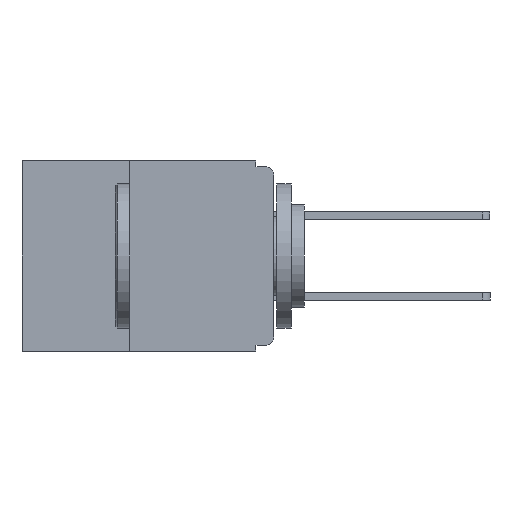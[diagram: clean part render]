
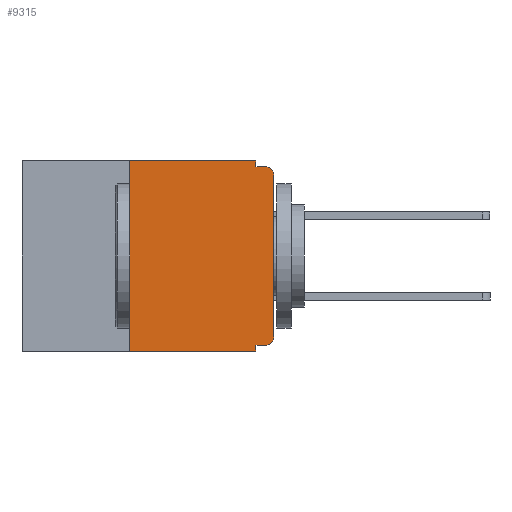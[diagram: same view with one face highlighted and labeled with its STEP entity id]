
A CAD part, left-side view. The second image highlights one B-rep face of the part: STEP entity #9315.
In plain terms, the highlighted planar face has unit normal (-1, 0, 0).
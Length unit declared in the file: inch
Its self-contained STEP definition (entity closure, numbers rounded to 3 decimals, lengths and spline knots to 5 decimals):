
#1121 = EDGE_CURVE ( 'NONE', #32581, #34202, #26190, .T. ) ;
#1328 = ORIENTED_EDGE ( 'NONE', *, *, #6280, .T. ) ;
#1453 = LINE ( 'NONE', #19023, #15636 ) ;
#1530 = EDGE_CURVE ( 'NONE', #34202, #16824, #20621, .T. ) ;
#2243 = ORIENTED_EDGE ( 'NONE', *, *, #1530, .F. ) ;
#2253 = LINE ( 'NONE', #21068, #15534 ) ;
#2695 = ORIENTED_EDGE ( 'NONE', *, *, #3785, .F. ) ;
#3785 = EDGE_CURVE ( 'NONE', #26825, #7777, #22980, .T. ) ;
#5232 = CARTESIAN_POINT ( 'NONE',  ( 0., 0.015, -0.01 ) ) ;
#5773 = ORIENTED_EDGE ( 'NONE', *, *, #33446, .F. ) ;
#6280 = EDGE_CURVE ( 'NONE', #29298, #16824, #17325, .T. ) ;
#6880 = CARTESIAN_POINT ( 'NONE',  ( 0., 0.031, -0.33 ) ) ;
#7129 = CIRCLE ( 'NONE', #20859, 0.015 ) ;
#7777 = VERTEX_POINT ( 'NONE', #15712 ) ;
#7837 = DIRECTION ( 'NONE',  ( 0., 0., -1. ) ) ;
#7987 = ORIENTED_EDGE ( 'NONE', *, *, #27274, .T. ) ;
#8113 = VECTOR ( 'NONE', #19153, 39.37008 ) ;
#8131 = DIRECTION ( 'NONE',  ( 0., -1., 0. ) ) ;
#8909 = CARTESIAN_POINT ( 'NONE',  ( 0., 0.25, -0.33 ) ) ;
#9092 = VECTOR ( 'NONE', #25122, 39.37008 ) ;
#9315 = ADVANCED_FACE ( 'NONE', ( #35630 ), #28338, .F. ) ;
#10619 = VECTOR ( 'NONE', #35682, 39.37008 ) ;
#10655 = ORIENTED_EDGE ( 'NONE', *, *, #1121, .F. ) ;
#11021 = EDGE_CURVE ( 'NONE', #7777, #24687, #1453, .T. ) ;
#11680 = DIRECTION ( 'NONE',  ( 0., -1., 0. ) ) ;
#11895 = DIRECTION ( 'NONE',  ( 1., 0., 0. ) ) ;
#12421 = DIRECTION ( 'NONE',  ( 0., 0., -1. ) ) ;
#12433 = DIRECTION ( 'NONE',  ( -1., 0., 0. ) ) ;
#12469 = CARTESIAN_POINT ( 'NONE',  ( 0., 0.015, -0.025 ) ) ;
#12589 = AXIS2_PLACEMENT_3D ( 'NONE', #12469, #12433, #12421 ) ;
#12830 = VERTEX_POINT ( 'NONE', #23644 ) ;
#12970 = CARTESIAN_POINT ( 'NONE',  ( 0., 0.015, -0.305 ) ) ;
#14036 = VECTOR ( 'NONE', #19601, 39.37008 ) ;
#15020 = AXIS2_PLACEMENT_3D ( 'NONE', #22870, #11895, #31139 ) ;
#15534 = VECTOR ( 'NONE', #26709, 39.37008 ) ;
#15636 = VECTOR ( 'NONE', #7837, 39.37008 ) ;
#15712 = CARTESIAN_POINT ( 'NONE',  ( 0., 0.031, -0.32 ) ) ;
#15819 = DIRECTION ( 'NONE',  ( 0., 0., -1. ) ) ;
#16824 = VERTEX_POINT ( 'NONE', #5232 ) ;
#16826 = CARTESIAN_POINT ( 'NONE',  ( 0., 0.437, -0.33 ) ) ;
#16848 = ORIENTED_EDGE ( 'NONE', *, *, #11021, .F. ) ;
#17325 = CIRCLE ( 'NONE', #12589, 0.015 ) ;
#17557 = CARTESIAN_POINT ( 'NONE',  ( 0., 0.437, 0. ) ) ;
#18570 = ORIENTED_EDGE ( 'NONE', *, *, #34724, .T. ) ;
#18919 = VECTOR ( 'NONE', #8131, 39.37008 ) ;
#19023 = CARTESIAN_POINT ( 'NONE',  ( 0., 0.031, -0.33 ) ) ;
#19153 = DIRECTION ( 'NONE',  ( 0., 0., 1. ) ) ;
#19218 = CARTESIAN_POINT ( 'NONE',  ( 0., 0.015, -0.32 ) ) ;
#19601 = DIRECTION ( 'NONE',  ( 0., -1., 0. ) ) ;
#20621 = LINE ( 'NONE', #29632, #18919 ) ;
#20859 = AXIS2_PLACEMENT_3D ( 'NONE', #12970, #32166, #15819 ) ;
#20860 = CARTESIAN_POINT ( 'NONE',  ( 0., 0.031, 0. ) ) ;
#21068 = CARTESIAN_POINT ( 'NONE',  ( 0., 0., 0. ) ) ;
#21453 = VECTOR ( 'NONE', #11680, 39.37008 ) ;
#21874 = CARTESIAN_POINT ( 'NONE',  ( 0., 0.25, -0.33 ) ) ;
#22304 = LINE ( 'NONE', #17557, #21453 ) ;
#22381 = ORIENTED_EDGE ( 'NONE', *, *, #29952, .T. ) ;
#22870 = CARTESIAN_POINT ( 'NONE',  ( 0., 0.437, 0. ) ) ;
#22900 = LINE ( 'NONE', #21874, #8113 ) ;
#22980 = LINE ( 'NONE', #24316, #9092 ) ;
#23644 = CARTESIAN_POINT ( 'NONE',  ( 0., 0.25, 0. ) ) ;
#24316 = CARTESIAN_POINT ( 'NONE',  ( 0., 0., -0.32 ) ) ;
#24687 = VERTEX_POINT ( 'NONE', #6880 ) ;
#25122 = DIRECTION ( 'NONE',  ( 0., 1., 0. ) ) ;
#26088 = CARTESIAN_POINT ( 'NONE',  ( 0., 0., -0.305 ) ) ;
#26190 = LINE ( 'NONE', #35369, #10619 ) ;
#26709 = DIRECTION ( 'NONE',  ( 0., 0., 1. ) ) ;
#26825 = VERTEX_POINT ( 'NONE', #19218 ) ;
#27110 = ORIENTED_EDGE ( 'NONE', *, *, #35691, .F. ) ;
#27274 = EDGE_CURVE ( 'NONE', #29018, #29298, #2253, .T. ) ;
#28338 = PLANE ( 'NONE',  #15020 ) ;
#29018 = VERTEX_POINT ( 'NONE', #26088 ) ;
#29298 = VERTEX_POINT ( 'NONE', #32819 ) ;
#29632 = CARTESIAN_POINT ( 'NONE',  ( 0., 0., -0.01 ) ) ;
#29952 = EDGE_CURVE ( 'NONE', #30063, #24687, #30389, .T. ) ;
#30063 = VERTEX_POINT ( 'NONE', #8909 ) ;
#30389 = LINE ( 'NONE', #16826, #14036 ) ;
#30683 = CARTESIAN_POINT ( 'NONE',  ( 0., 0.031, -0.01 ) ) ;
#31139 = DIRECTION ( 'NONE',  ( 0., 0., -1. ) ) ;
#32166 = DIRECTION ( 'NONE',  ( -1., 0., 0. ) ) ;
#32338 = EDGE_LOOP ( 'NONE', ( #7987, #1328, #2243, #10655, #27110, #5773, #22381, #16848, #2695, #18570 ) ) ;
#32581 = VERTEX_POINT ( 'NONE', #20860 ) ;
#32819 = CARTESIAN_POINT ( 'NONE',  ( 0., 0., -0.025 ) ) ;
#33446 = EDGE_CURVE ( 'NONE', #30063, #12830, #22900, .T. ) ;
#34202 = VERTEX_POINT ( 'NONE', #30683 ) ;
#34724 = EDGE_CURVE ( 'NONE', #26825, #29018, #7129, .T. ) ;
#35369 = CARTESIAN_POINT ( 'NONE',  ( 0., 0.031, 0. ) ) ;
#35630 = FACE_OUTER_BOUND ( 'NONE', #32338, .T. ) ;
#35682 = DIRECTION ( 'NONE',  ( 0., 0., -1. ) ) ;
#35691 = EDGE_CURVE ( 'NONE', #12830, #32581, #22304, .T. ) ;
